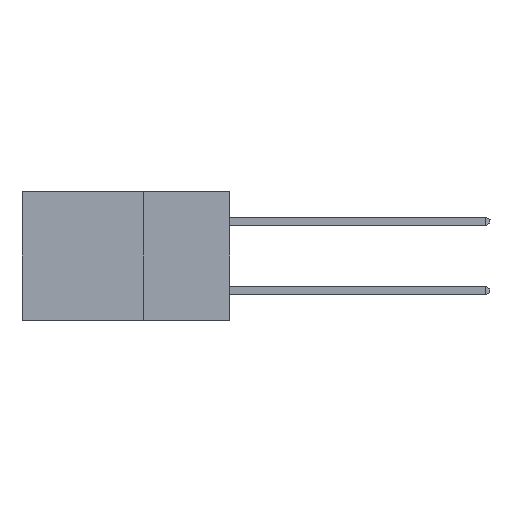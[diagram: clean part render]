
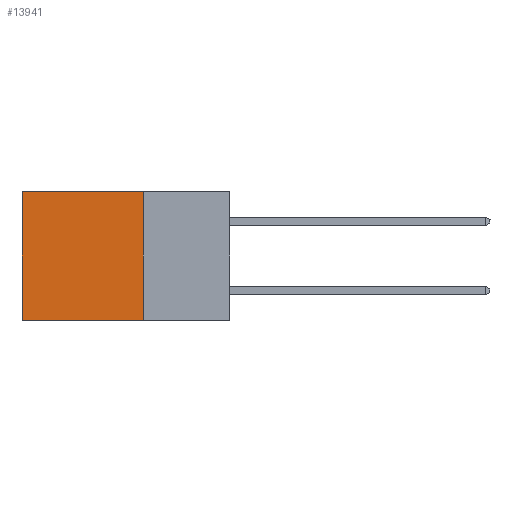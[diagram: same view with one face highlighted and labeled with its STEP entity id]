
A CAD part, left-side view. The second image highlights one B-rep face of the part: STEP entity #13941.
In plain terms, the highlighted planar face has unit normal (-1, 0, 0).
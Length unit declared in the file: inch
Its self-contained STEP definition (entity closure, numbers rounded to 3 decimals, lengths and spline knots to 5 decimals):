
#91 = CARTESIAN_POINT ( 'NONE',  ( 0.298, 0.25, 0. ) ) ;
#895 = DIRECTION ( 'NONE',  ( 1., 0., 0. ) ) ;
#1240 = VECTOR ( 'NONE', #1907, 39.37008 ) ;
#1621 = EDGE_CURVE ( 'NONE', #7529, #11251, #16736, .T. ) ;
#1646 = CARTESIAN_POINT ( 'NONE',  ( 0.298, 0.6, -0.37 ) ) ;
#1781 = VERTEX_POINT ( 'NONE', #17579 ) ;
#1907 = DIRECTION ( 'NONE',  ( 0., 0., -1. ) ) ;
#2253 = CARTESIAN_POINT ( 'NONE',  ( 0.298, 0.25, 0. ) ) ;
#2439 = VECTOR ( 'NONE', #7120, 39.37008 ) ;
#2466 = EDGE_CURVE ( 'NONE', #2665, #1781, #4315, .T. ) ;
#2665 = VERTEX_POINT ( 'NONE', #91 ) ;
#2767 = EDGE_CURVE ( 'NONE', #2665, #7529, #15962, .T. ) ;
#3285 = CARTESIAN_POINT ( 'NONE',  ( 0.298, 0.6, 0. ) ) ;
#3586 = ORIENTED_EDGE ( 'NONE', *, *, #2466, .F. ) ;
#4094 = EDGE_CURVE ( 'NONE', #1781, #11251, #15035, .T. ) ;
#4295 = CARTESIAN_POINT ( 'NONE',  ( 0.298, 0.25, -0.37 ) ) ;
#4315 = LINE ( 'NONE', #15054, #9841 ) ;
#5245 = PLANE ( 'NONE',  #8166 ) ;
#5580 = VECTOR ( 'NONE', #15726, 39.37008 ) ;
#7120 = DIRECTION ( 'NONE',  ( 0., 1., 0. ) ) ;
#7529 = VERTEX_POINT ( 'NONE', #10538 ) ;
#8166 = AXIS2_PLACEMENT_3D ( 'NONE', #2253, #895, #13604 ) ;
#9841 = VECTOR ( 'NONE', #13685, 39.37008 ) ;
#10538 = CARTESIAN_POINT ( 'NONE',  ( 0.298, 0.6, 0. ) ) ;
#11251 = VERTEX_POINT ( 'NONE', #1646 ) ;
#12895 = EDGE_LOOP ( 'NONE', ( #16749, #17565, #3586, #18265 ) ) ;
#13604 = DIRECTION ( 'NONE',  ( 0., 0., -1. ) ) ;
#13685 = DIRECTION ( 'NONE',  ( 0., 0., -1. ) ) ;
#13941 = ADVANCED_FACE ( 'NONE', ( #15627 ), #5245, .F. ) ;
#15035 = LINE ( 'NONE', #4295, #2439 ) ;
#15054 = CARTESIAN_POINT ( 'NONE',  ( 0.298, 0.25, 0. ) ) ;
#15627 = FACE_OUTER_BOUND ( 'NONE', #12895, .T. ) ;
#15726 = DIRECTION ( 'NONE',  ( 0., 1., 0. ) ) ;
#15962 = LINE ( 'NONE', #17247, #5580 ) ;
#16736 = LINE ( 'NONE', #3285, #1240 ) ;
#16749 = ORIENTED_EDGE ( 'NONE', *, *, #1621, .T. ) ;
#17247 = CARTESIAN_POINT ( 'NONE',  ( 0.298, 0.25, 0. ) ) ;
#17565 = ORIENTED_EDGE ( 'NONE', *, *, #4094, .F. ) ;
#17579 = CARTESIAN_POINT ( 'NONE',  ( 0.298, 0.25, -0.37 ) ) ;
#18265 = ORIENTED_EDGE ( 'NONE', *, *, #2767, .T. ) ;
